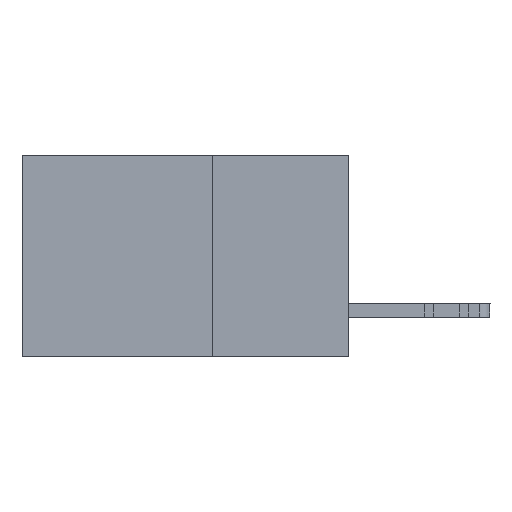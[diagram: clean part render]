
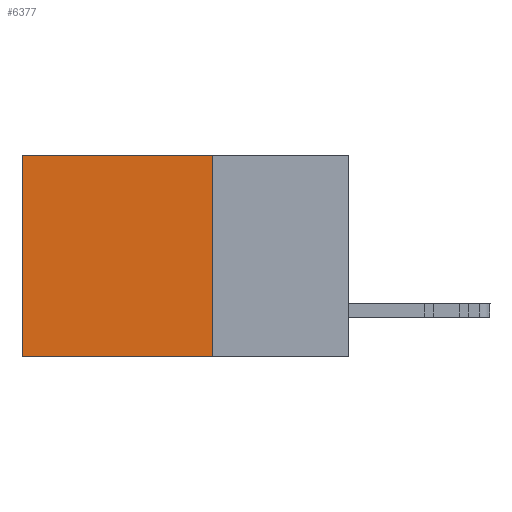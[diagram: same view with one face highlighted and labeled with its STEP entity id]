
A CAD part, left-side view. The second image highlights one B-rep face of the part: STEP entity #6377.
In plain terms, the highlighted planar face has unit normal (-1, 0, 0).
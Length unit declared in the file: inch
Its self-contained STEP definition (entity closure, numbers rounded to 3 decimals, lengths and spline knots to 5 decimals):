
#55 = DIRECTION ( 'NONE',  ( 1., 0., 0. ) ) ;
#573 = ORIENTED_EDGE ( 'NONE', *, *, #20170, .F. ) ;
#1184 = CARTESIAN_POINT ( 'NONE',  ( 0.2615, 0.25, 0. ) ) ;
#1404 = CARTESIAN_POINT ( 'NONE',  ( 0.2615, 0.25, -0.37 ) ) ;
#1578 = CARTESIAN_POINT ( 'NONE',  ( 0.2615, 0.6, 0. ) ) ;
#1723 = VECTOR ( 'NONE', #23135, 39.37008 ) ;
#1775 = CARTESIAN_POINT ( 'NONE',  ( 0.2615, 0.6, -0.37 ) ) ;
#2066 = CARTESIAN_POINT ( 'NONE',  ( 0.2615, 0.25, -0.37 ) ) ;
#3317 = LINE ( 'NONE', #18161, #9149 ) ;
#5037 = EDGE_LOOP ( 'NONE', ( #16463, #12972, #573, #8808 ) ) ;
#5433 = VERTEX_POINT ( 'NONE', #1184 ) ;
#5534 = DIRECTION ( 'NONE',  ( 0., 1., 0. ) ) ;
#6377 = ADVANCED_FACE ( 'NONE', ( #21176 ), #13523, .F. ) ;
#6670 = DIRECTION ( 'NONE',  ( 0., 0., -1. ) ) ;
#7757 = LINE ( 'NONE', #1404, #13459 ) ;
#7831 = EDGE_CURVE ( 'NONE', #22042, #21483, #3317, .T. ) ;
#8808 = ORIENTED_EDGE ( 'NONE', *, *, #20036, .T. ) ;
#9149 = VECTOR ( 'NONE', #6670, 39.37008 ) ;
#12972 = ORIENTED_EDGE ( 'NONE', *, *, #21998, .F. ) ;
#13237 = CARTESIAN_POINT ( 'NONE',  ( 0.2615, 0.25, 0. ) ) ;
#13459 = VECTOR ( 'NONE', #16895, 39.37008 ) ;
#13523 = PLANE ( 'NONE',  #24507 ) ;
#13602 = DIRECTION ( 'NONE',  ( 0., 0., -1. ) ) ;
#14459 = LINE ( 'NONE', #13237, #23980 ) ;
#16463 = ORIENTED_EDGE ( 'NONE', *, *, #7831, .T. ) ;
#16563 = LINE ( 'NONE', #21245, #1723 ) ;
#16895 = DIRECTION ( 'NONE',  ( 0., 1., 0. ) ) ;
#18161 = CARTESIAN_POINT ( 'NONE',  ( 0.2615, 0.6, -0.37 ) ) ;
#19492 = CARTESIAN_POINT ( 'NONE',  ( 0.2615, 0.25, -0.37 ) ) ;
#19974 = VERTEX_POINT ( 'NONE', #2066 ) ;
#20036 = EDGE_CURVE ( 'NONE', #5433, #22042, #14459, .T. ) ;
#20170 = EDGE_CURVE ( 'NONE', #5433, #19974, #16563, .T. ) ;
#21176 = FACE_OUTER_BOUND ( 'NONE', #5037, .T. ) ;
#21245 = CARTESIAN_POINT ( 'NONE',  ( 0.2615, 0.25, -0.37 ) ) ;
#21483 = VERTEX_POINT ( 'NONE', #1775 ) ;
#21998 = EDGE_CURVE ( 'NONE', #19974, #21483, #7757, .T. ) ;
#22042 = VERTEX_POINT ( 'NONE', #1578 ) ;
#23135 = DIRECTION ( 'NONE',  ( 0., 0., -1. ) ) ;
#23980 = VECTOR ( 'NONE', #5534, 39.37008 ) ;
#24507 = AXIS2_PLACEMENT_3D ( 'NONE', #19492, #55, #13602 ) ;
